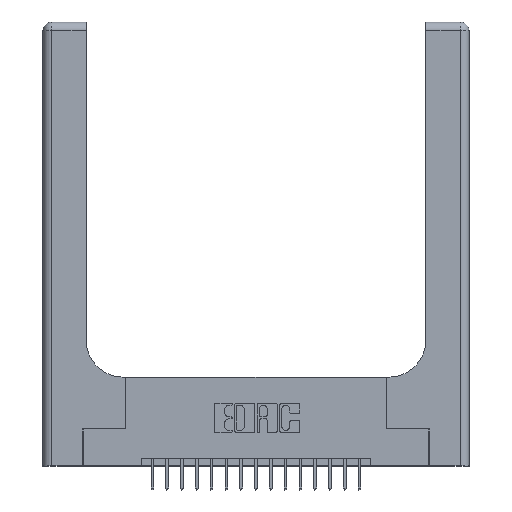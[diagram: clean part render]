
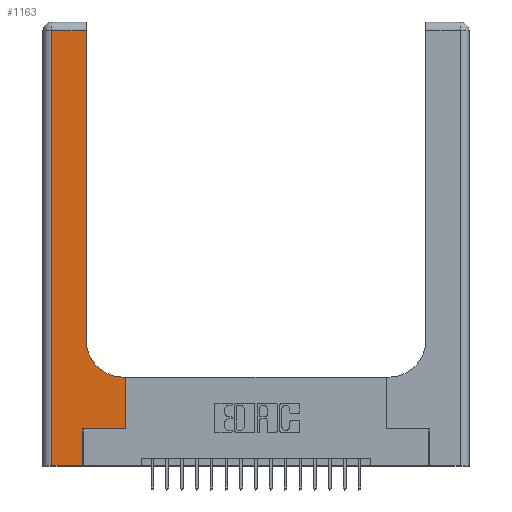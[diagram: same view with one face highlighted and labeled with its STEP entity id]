
A CAD part, top view. The second image highlights one B-rep face of the part: STEP entity #1163.
In plain terms, the highlighted planar face has unit normal (0, 0, 1).
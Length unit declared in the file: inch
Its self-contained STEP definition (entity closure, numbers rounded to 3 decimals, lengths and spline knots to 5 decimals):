
#536 = ORIENTED_EDGE ( 'NONE', *, *, #8589, .T. ) ;
#650 = EDGE_LOOP ( 'NONE', ( #7771, #2639, #536, #11303, #18116, #5511, #18660, #16539, #1613 ) ) ;
#1163 = ADVANCED_FACE ( 'NONE', ( #14521 ), #1679, .F. ) ;
#1613 = ORIENTED_EDGE ( 'NONE', *, *, #15929, .T. ) ;
#1676 = VECTOR ( 'NONE', #11004, 39.37008 ) ;
#1679 = PLANE ( 'NONE',  #7216 ) ;
#1999 = DIRECTION ( 'NONE',  ( 0., -1., 0. ) ) ;
#2161 = DIRECTION ( 'NONE',  ( -1., 0., 0. ) ) ;
#2162 = CARTESIAN_POINT ( 'NONE',  ( 0.5585, 0.6, 0.37 ) ) ;
#2315 = CARTESIAN_POINT ( 'NONE',  ( 0.06, 0., 0.37 ) ) ;
#2518 = CARTESIAN_POINT ( 'NONE',  ( 0.5585, 0.25, 0.37 ) ) ;
#2618 = CARTESIAN_POINT ( 'NONE',  ( 0., 0., 0.37 ) ) ;
#2639 = ORIENTED_EDGE ( 'NONE', *, *, #17398, .T. ) ;
#3069 = VERTEX_POINT ( 'NONE', #2315 ) ;
#3186 = DIRECTION ( 'NONE',  ( -1., 0., 0. ) ) ;
#3502 = EDGE_CURVE ( 'NONE', #18714, #10058, #15381, .T. ) ;
#3690 = VERTEX_POINT ( 'NONE', #10529 ) ;
#3727 = DIRECTION ( 'NONE',  ( 0., 1., 0. ) ) ;
#3800 = CARTESIAN_POINT ( 'NONE',  ( 0.5415, 0.6, 0.37 ) ) ;
#3843 = VECTOR ( 'NONE', #18679, 39.37008 ) ;
#4039 = LINE ( 'NONE', #14896, #5782 ) ;
#4298 = DIRECTION ( 'NONE',  ( 1., 0., 0. ) ) ;
#5511 = ORIENTED_EDGE ( 'NONE', *, *, #8043, .T. ) ;
#5754 = DIRECTION ( 'NONE',  ( 0., 1., 0. ) ) ;
#5782 = VECTOR ( 'NONE', #1999, 39.37008 ) ;
#5915 = LINE ( 'NONE', #2618, #14853 ) ;
#6509 = CARTESIAN_POINT ( 'NONE',  ( 0.06, 2.94, 0.37 ) ) ;
#7216 = AXIS2_PLACEMENT_3D ( 'NONE', #17521, #19185, #2161 ) ;
#7373 = LINE ( 'NONE', #2518, #12127 ) ;
#7510 = EDGE_CURVE ( 'NONE', #11268, #19120, #13053, .T. ) ;
#7538 = CARTESIAN_POINT ( 'NONE',  ( 0.269, 0.25, 0.37 ) ) ;
#7632 = DIRECTION ( 'NONE',  ( 1., 0., 0. ) ) ;
#7771 = ORIENTED_EDGE ( 'NONE', *, *, #16346, .T. ) ;
#8043 = EDGE_CURVE ( 'NONE', #10058, #18775, #13779, .T. ) ;
#8317 = CARTESIAN_POINT ( 'NONE',  ( 0.269, 0., 0.37 ) ) ;
#8589 = EDGE_CURVE ( 'NONE', #18088, #3069, #4039, .T. ) ;
#9162 = CARTESIAN_POINT ( 'NONE',  ( 0.2915, 0.6, 0.37 ) ) ;
#10058 = VERTEX_POINT ( 'NONE', #7538 ) ;
#10529 = CARTESIAN_POINT ( 'NONE',  ( 0.2915, 0.85, 0.37 ) ) ;
#11004 = DIRECTION ( 'NONE',  ( 0., 1., 0. ) ) ;
#11017 = DIRECTION ( 'NONE',  ( 0., 0., -1. ) ) ;
#11268 = VERTEX_POINT ( 'NONE', #2162 ) ;
#11303 = ORIENTED_EDGE ( 'NONE', *, *, #17221, .T. ) ;
#12127 = VECTOR ( 'NONE', #5754, 39.37008 ) ;
#12602 = CARTESIAN_POINT ( 'NONE',  ( 0.5585, 0.25, 0.37 ) ) ;
#13053 = LINE ( 'NONE', #9162, #3843 ) ;
#13779 = LINE ( 'NONE', #18970, #19017 ) ;
#14325 = AXIS2_PLACEMENT_3D ( 'NONE', #18951, #11017, #17937 ) ;
#14521 = FACE_OUTER_BOUND ( 'NONE', #650, .T. ) ;
#14839 = VERTEX_POINT ( 'NONE', #15074 ) ;
#14853 = VECTOR ( 'NONE', #4298, 39.37008 ) ;
#14896 = CARTESIAN_POINT ( 'NONE',  ( 0.06, 3., 0.37 ) ) ;
#15074 = CARTESIAN_POINT ( 'NONE',  ( 0.2915, 2.94, 0.37 ) ) ;
#15096 = CARTESIAN_POINT ( 'NONE',  ( 0.269, 0., 0.37 ) ) ;
#15381 = LINE ( 'NONE', #8317, #17908 ) ;
#15602 = LINE ( 'NONE', #19260, #16115 ) ;
#15929 = EDGE_CURVE ( 'NONE', #19120, #3690, #19662, .T. ) ;
#16115 = VECTOR ( 'NONE', #3186, 39.37008 ) ;
#16346 = EDGE_CURVE ( 'NONE', #3690, #14839, #20145, .T. ) ;
#16539 = ORIENTED_EDGE ( 'NONE', *, *, #7510, .T. ) ;
#17221 = EDGE_CURVE ( 'NONE', #3069, #18714, #5915, .T. ) ;
#17398 = EDGE_CURVE ( 'NONE', #14839, #18088, #15602, .T. ) ;
#17521 = CARTESIAN_POINT ( 'NONE',  ( 0., 3., 0.37 ) ) ;
#17673 = EDGE_CURVE ( 'NONE', #18775, #11268, #7373, .T. ) ;
#17908 = VECTOR ( 'NONE', #3727, 39.37008 ) ;
#17937 = DIRECTION ( 'NONE',  ( 1., 0., 0. ) ) ;
#18088 = VERTEX_POINT ( 'NONE', #6509 ) ;
#18116 = ORIENTED_EDGE ( 'NONE', *, *, #3502, .T. ) ;
#18660 = ORIENTED_EDGE ( 'NONE', *, *, #17673, .T. ) ;
#18679 = DIRECTION ( 'NONE',  ( -1., 0., 0. ) ) ;
#18714 = VERTEX_POINT ( 'NONE', #15096 ) ;
#18775 = VERTEX_POINT ( 'NONE', #12602 ) ;
#18951 = CARTESIAN_POINT ( 'NONE',  ( 0.5415, 0.85, 0.37 ) ) ;
#18970 = CARTESIAN_POINT ( 'NONE',  ( 0.269, 0.25, 0.37 ) ) ;
#19017 = VECTOR ( 'NONE', #7632, 39.37008 ) ;
#19120 = VERTEX_POINT ( 'NONE', #3800 ) ;
#19185 = DIRECTION ( 'NONE',  ( 0., 0., -1. ) ) ;
#19260 = CARTESIAN_POINT ( 'NONE',  ( 0., 2.94, 0.37 ) ) ;
#19662 = CIRCLE ( 'NONE', #14325, 0.25 ) ;
#20145 = LINE ( 'NONE', #20400, #1676 ) ;
#20400 = CARTESIAN_POINT ( 'NONE',  ( 0.2915, 3., 0.37 ) ) ;
